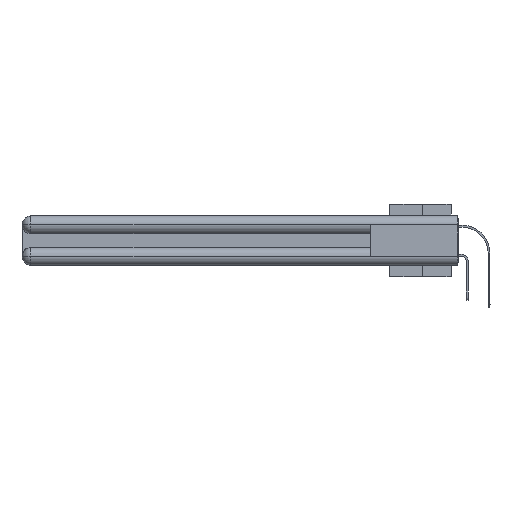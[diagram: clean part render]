
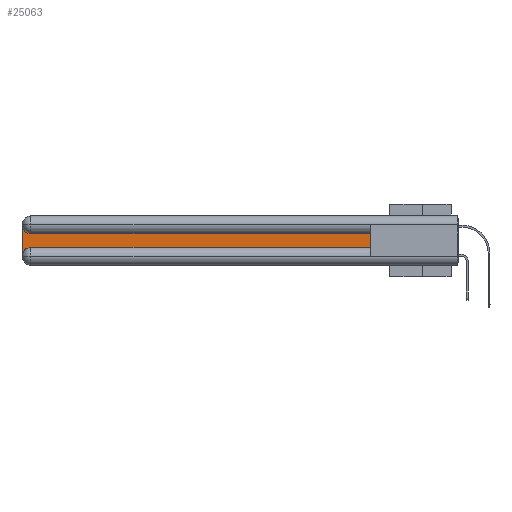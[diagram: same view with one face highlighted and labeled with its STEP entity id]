
A CAD part, left-side view. The second image highlights one B-rep face of the part: STEP entity #25063.
In plain terms, the highlighted planar face has unit normal (-1, 0, 0).
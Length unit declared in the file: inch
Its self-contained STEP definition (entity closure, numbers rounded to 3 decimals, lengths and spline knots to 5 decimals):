
#705 = VECTOR ( 'NONE', #23854, 39.37008 ) ;
#1119 = LINE ( 'NONE', #19014, #705 ) ;
#3089 = LINE ( 'NONE', #30830, #7866 ) ;
#4736 = EDGE_CURVE ( 'NONE', #32462, #14854, #1119, .T. ) ;
#4908 = ORIENTED_EDGE ( 'NONE', *, *, #20005, .T. ) ;
#6034 = ORIENTED_EDGE ( 'NONE', *, *, #30157, .T. ) ;
#6180 = CARTESIAN_POINT ( 'NONE',  ( 0.075, 2.94, -0.2775 ) ) ;
#7866 = VECTOR ( 'NONE', #27988, 39.37008 ) ;
#8024 = PLANE ( 'NONE',  #14466 ) ;
#8059 = VERTEX_POINT ( 'NONE', #29479 ) ;
#8784 = DIRECTION ( 'NONE',  ( 1., 0., 0. ) ) ;
#9137 = EDGE_CURVE ( 'NONE', #14854, #21020, #3089, .T. ) ;
#10364 = DIRECTION ( 'NONE',  ( 0., -1., 0. ) ) ;
#10536 = FACE_OUTER_BOUND ( 'NONE', #24471, .T. ) ;
#10855 = DIRECTION ( 'NONE',  ( 0., 0., -1. ) ) ;
#11116 = VERTEX_POINT ( 'NONE', #20058 ) ;
#11342 = CARTESIAN_POINT ( 'NONE',  ( 0.075, 3., -0.2775 ) ) ;
#12858 = ORIENTED_EDGE ( 'NONE', *, *, #4736, .T. ) ;
#12875 = DIRECTION ( 'NONE',  ( 1., 0., 0. ) ) ;
#14466 = AXIS2_PLACEMENT_3D ( 'NONE', #20746, #12875, #27907 ) ;
#14600 = CARTESIAN_POINT ( 'NONE',  ( 0.075, 0.6, -0.2175 ) ) ;
#14854 = VERTEX_POINT ( 'NONE', #30860 ) ;
#16360 = DIRECTION ( 'NONE',  ( 1., 0., 0. ) ) ;
#17366 = AXIS2_PLACEMENT_3D ( 'NONE', #31680, #8784, #18825 ) ;
#18825 = DIRECTION ( 'NONE',  ( 0., 0., -1. ) ) ;
#19014 = CARTESIAN_POINT ( 'NONE',  ( 0.075, 0.6, -0.2175 ) ) ;
#20005 = EDGE_CURVE ( 'NONE', #11116, #32462, #22900, .T. ) ;
#20045 = ORIENTED_EDGE ( 'NONE', *, *, #9137, .T. ) ;
#20058 = CARTESIAN_POINT ( 'NONE',  ( 0.075, 2.94, -0.2175 ) ) ;
#20169 = EDGE_CURVE ( 'NONE', #29635, #11116, #32863, .T. ) ;
#20390 = CARTESIAN_POINT ( 'NONE',  ( 0.075, 0.6, -0.2175 ) ) ;
#20645 = CARTESIAN_POINT ( 'NONE',  ( 0.075, 2.94, -0.1225 ) ) ;
#20746 = CARTESIAN_POINT ( 'NONE',  ( 0.075, 3., -0.1225 ) ) ;
#21020 = VERTEX_POINT ( 'NONE', #20645 ) ;
#22900 = LINE ( 'NONE', #14600, #27042 ) ;
#23395 = CARTESIAN_POINT ( 'NONE',  ( 0.075, 3., -0.2175 ) ) ;
#23854 = DIRECTION ( 'NONE',  ( 0., 0., 1. ) ) ;
#24290 = CIRCLE ( 'NONE', #17366, 0.06 ) ;
#24471 = EDGE_LOOP ( 'NONE', ( #20045, #6034, #31366, #30660, #4908, #12858 ) ) ;
#24564 = VECTOR ( 'NONE', #10855, 39.37008 ) ;
#25063 = ADVANCED_FACE ( 'NONE', ( #10536 ), #8024, .F. ) ;
#26189 = EDGE_CURVE ( 'NONE', #8059, #29635, #28227, .T. ) ;
#26545 = DIRECTION ( 'NONE',  ( 0., 0., -1. ) ) ;
#27042 = VECTOR ( 'NONE', #10364, 39.37008 ) ;
#27907 = DIRECTION ( 'NONE',  ( 0., 0., -1. ) ) ;
#27988 = DIRECTION ( 'NONE',  ( 0., 1., 0. ) ) ;
#28227 = LINE ( 'NONE', #23395, #24564 ) ;
#29479 = CARTESIAN_POINT ( 'NONE',  ( 0.075, 3., -0.0625 ) ) ;
#29635 = VERTEX_POINT ( 'NONE', #11342 ) ;
#30157 = EDGE_CURVE ( 'NONE', #21020, #8059, #24290, .T. ) ;
#30660 = ORIENTED_EDGE ( 'NONE', *, *, #20169, .T. ) ;
#30830 = CARTESIAN_POINT ( 'NONE',  ( 0.075, 0.6, -0.1225 ) ) ;
#30860 = CARTESIAN_POINT ( 'NONE',  ( 0.075, 0.6, -0.1225 ) ) ;
#31366 = ORIENTED_EDGE ( 'NONE', *, *, #26189, .T. ) ;
#31680 = CARTESIAN_POINT ( 'NONE',  ( 0.075, 2.94, -0.0625 ) ) ;
#31863 = AXIS2_PLACEMENT_3D ( 'NONE', #6180, #16360, #26545 ) ;
#32462 = VERTEX_POINT ( 'NONE', #20390 ) ;
#32863 = CIRCLE ( 'NONE', #31863, 0.06 ) ;
